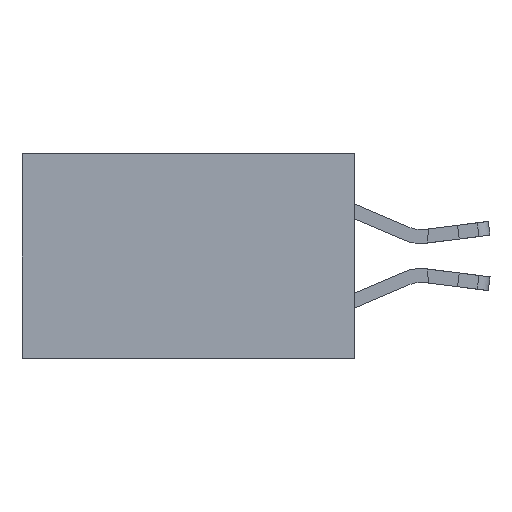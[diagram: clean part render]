
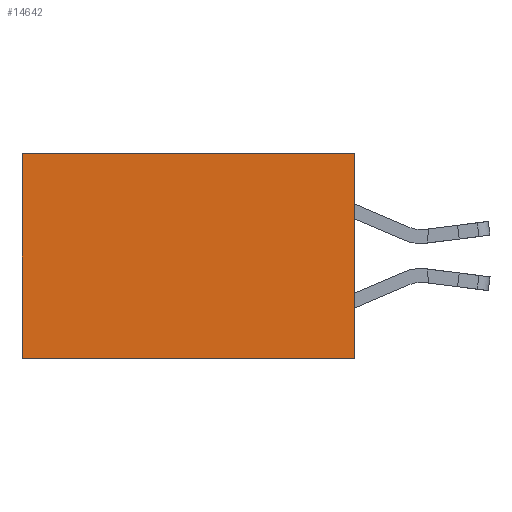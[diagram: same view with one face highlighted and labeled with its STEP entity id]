
A CAD part, left-side view. The second image highlights one B-rep face of the part: STEP entity #14642.
In plain terms, the highlighted planar face has unit normal (-1, 0, 0).
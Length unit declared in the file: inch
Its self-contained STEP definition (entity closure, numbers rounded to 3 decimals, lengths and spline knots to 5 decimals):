
#185 = DIRECTION ( 'NONE',  ( 0., 0., -1. ) ) ;
#213 = CARTESIAN_POINT ( 'NONE',  ( 0.2615, 0.6, -0.37 ) ) ;
#217 = DIRECTION ( 'NONE',  ( 1., 0., 0. ) ) ;
#288 = DIRECTION ( 'NONE',  ( 0., 1., 0. ) ) ;
#484 = EDGE_CURVE ( 'NONE', #6295, #15567, #15476, .T. ) ;
#623 = PLANE ( 'NONE',  #4258 ) ;
#787 = EDGE_CURVE ( 'NONE', #6295, #10977, #8568, .T. ) ;
#1074 = CARTESIAN_POINT ( 'NONE',  ( 0.2615, 0., -0.37 ) ) ;
#1209 = LINE ( 'NONE', #1074, #7601 ) ;
#1225 = CARTESIAN_POINT ( 'NONE',  ( 0.2615, 0., -0.37 ) ) ;
#2189 = DIRECTION ( 'NONE',  ( 0., 1., 0. ) ) ;
#3167 = VERTEX_POINT ( 'NONE', #8388 ) ;
#3230 = CARTESIAN_POINT ( 'NONE',  ( 0.2615, 0., 0. ) ) ;
#3720 = FACE_OUTER_BOUND ( 'NONE', #7143, .T. ) ;
#4258 = AXIS2_PLACEMENT_3D ( 'NONE', #1225, #217, #185 ) ;
#5410 = CARTESIAN_POINT ( 'NONE',  ( 0.2615, 0., -0.37 ) ) ;
#5899 = VECTOR ( 'NONE', #12671, 39.37008 ) ;
#6295 = VERTEX_POINT ( 'NONE', #3230 ) ;
#6993 = CARTESIAN_POINT ( 'NONE',  ( 0.2615, 0.6, 0. ) ) ;
#7143 = EDGE_LOOP ( 'NONE', ( #10232, #10299, #10956, #13918 ) ) ;
#7206 = CARTESIAN_POINT ( 'NONE',  ( 0.2615, 0., 0. ) ) ;
#7601 = VECTOR ( 'NONE', #288, 39.37008 ) ;
#8000 = EDGE_CURVE ( 'NONE', #10977, #3167, #9711, .T. ) ;
#8388 = CARTESIAN_POINT ( 'NONE',  ( 0.2615, 0.6, -0.37 ) ) ;
#8568 = LINE ( 'NONE', #7206, #14495 ) ;
#8963 = VECTOR ( 'NONE', #9309, 39.37008 ) ;
#9309 = DIRECTION ( 'NONE',  ( 0., 0., -1. ) ) ;
#9711 = LINE ( 'NONE', #213, #5899 ) ;
#10232 = ORIENTED_EDGE ( 'NONE', *, *, #8000, .T. ) ;
#10299 = ORIENTED_EDGE ( 'NONE', *, *, #12338, .F. ) ;
#10956 = ORIENTED_EDGE ( 'NONE', *, *, #484, .F. ) ;
#10977 = VERTEX_POINT ( 'NONE', #6993 ) ;
#12338 = EDGE_CURVE ( 'NONE', #15567, #3167, #1209, .T. ) ;
#12671 = DIRECTION ( 'NONE',  ( 0., 0., -1. ) ) ;
#13533 = CARTESIAN_POINT ( 'NONE',  ( 0.2615, 0., -0.37 ) ) ;
#13918 = ORIENTED_EDGE ( 'NONE', *, *, #787, .T. ) ;
#14495 = VECTOR ( 'NONE', #2189, 39.37008 ) ;
#14642 = ADVANCED_FACE ( 'NONE', ( #3720 ), #623, .F. ) ;
#15476 = LINE ( 'NONE', #5410, #8963 ) ;
#15567 = VERTEX_POINT ( 'NONE', #13533 ) ;
